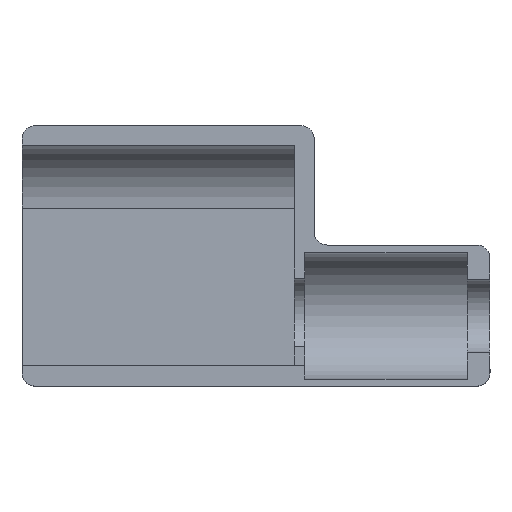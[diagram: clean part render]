
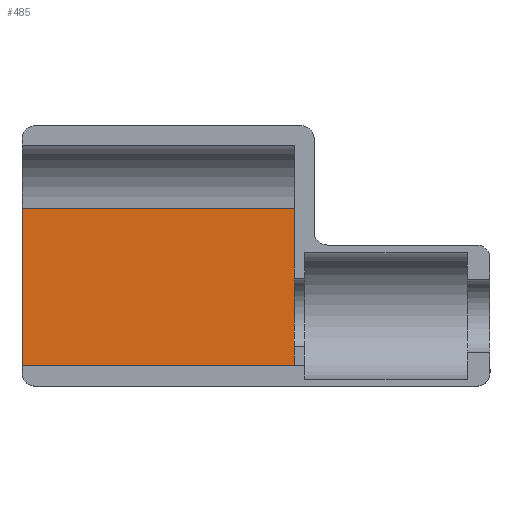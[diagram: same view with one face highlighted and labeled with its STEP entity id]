
A CAD part, top view. The second image highlights one B-rep face of the part: STEP entity #485.
In plain terms, the highlighted planar face has unit normal (0, 0, 1).
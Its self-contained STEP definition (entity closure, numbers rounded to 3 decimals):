
#30=PLANE('',#544);
#54=FACE_OUTER_BOUND('',#79,.T.);
#79=EDGE_LOOP('',(#427,#428,#429,#430));
#117=LINE('',#799,#166);
#118=LINE('',#803,#167);
#125=LINE('',#820,#174);
#126=LINE('',#822,#175);
#166=VECTOR('',#650,1000.);
#167=VECTOR('',#655,10.);
#174=VECTOR('',#672,10.);
#175=VECTOR('',#675,1000.);
#237=VERTEX_POINT('',#796);
#238=VERTEX_POINT('',#798);
#239=VERTEX_POINT('',#802);
#244=VERTEX_POINT('',#818);
#297=EDGE_CURVE('',#238,#237,#117,.T.);
#299=EDGE_CURVE('',#239,#238,#118,.T.);
#308=EDGE_CURVE('',#237,#244,#125,.T.);
#309=EDGE_CURVE('',#244,#239,#126,.T.);
#427=ORIENTED_EDGE('',*,*,#309,.T.);
#428=ORIENTED_EDGE('',*,*,#299,.T.);
#429=ORIENTED_EDGE('',*,*,#297,.T.);
#430=ORIENTED_EDGE('',*,*,#308,.T.);
#485=ADVANCED_FACE('',(#54),#30,.F.);
#544=AXIS2_PLACEMENT_3D('',#828,#679,#680);
#650=DIRECTION('',(-1.,0.,0.));
#655=DIRECTION('',(0.,1.,0.));
#672=DIRECTION('',(0.,-1.,0.));
#675=DIRECTION('',(1.,0.,0.));
#679=DIRECTION('center_axis',(0.,0.,
-1.));
#680=DIRECTION('ref_axis',(-1.,0.,0.));
#796=CARTESIAN_POINT('',(-52.381,10.705,6.));
#798=CARTESIAN_POINT('',(8.536,10.705,6.));
#799=CARTESIAN_POINT('',(7.681,10.705,6.));
#802=CARTESIAN_POINT('',(8.536,-24.495,6.));
#803=CARTESIAN_POINT('',(8.536,-26.577,6.));
#818=CARTESIAN_POINT('',(-52.381,-24.495,6.));
#820=CARTESIAN_POINT('',(-52.381,6.495,6.));
#822=CARTESIAN_POINT('',(-167.319,-24.495,6.));
#828=CARTESIAN_POINT('Origin',(7.681,-30.845,6.));
